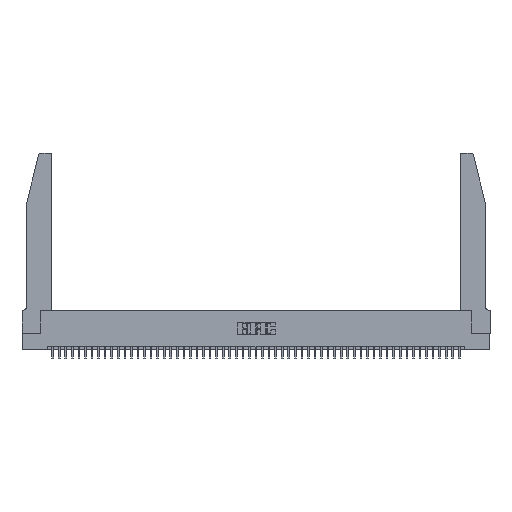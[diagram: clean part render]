
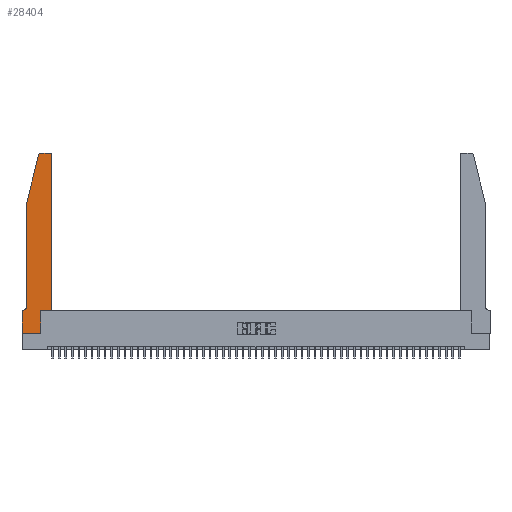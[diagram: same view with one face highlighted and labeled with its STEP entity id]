
A CAD part, top view. The second image highlights one B-rep face of the part: STEP entity #28404.
In plain terms, the highlighted planar face has unit normal (0, 0, 1).
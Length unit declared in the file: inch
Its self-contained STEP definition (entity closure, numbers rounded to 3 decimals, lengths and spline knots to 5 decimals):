
#653 = AXIS2_PLACEMENT_3D ( 'NONE', #5602, #33332, #9619 ) ;
#701 = CIRCLE ( 'NONE', #653, 0.03 ) ;
#879 = VERTEX_POINT ( 'NONE', #44375 ) ;
#1047 = DIRECTION ( 'NONE',  ( 0., -1., 0. ) ) ;
#1328 = VERTEX_POINT ( 'NONE', #31188 ) ;
#2118 = VERTEX_POINT ( 'NONE', #18137 ) ;
#2484 = CARTESIAN_POINT ( 'NONE',  ( 0.0755, 0.42, 0.37 ) ) ;
#4215 = CARTESIAN_POINT ( 'NONE',  ( 0.4205, 2.75, 0.37 ) ) ;
#4865 = CARTESIAN_POINT ( 'NONE',  ( 0., 0., 0.37 ) ) ;
#5602 = CARTESIAN_POINT ( 'NONE',  ( 0.284, 2.72, 0.37 ) ) ;
#5902 = ORIENTED_EDGE ( 'NONE', *, *, #31229, .T. ) ;
#6054 = ORIENTED_EDGE ( 'NONE', *, *, #18705, .T. ) ;
#6133 = VECTOR ( 'NONE', #19532, 39.37008 ) ;
#6512 = DIRECTION ( 'NONE',  ( 0., -1., 0. ) ) ;
#6820 = CARTESIAN_POINT ( 'NONE',  ( 0.4505, 0.35, 0.37 ) ) ;
#6958 = EDGE_CURVE ( 'NONE', #16118, #26908, #17446, .T. ) ;
#7067 = PLANE ( 'NONE',  #27129 ) ;
#7521 = DIRECTION ( 'NONE',  ( -0.239, -0.971, 0. ) ) ;
#7582 = CARTESIAN_POINT ( 'NONE',  ( 0.2865, 0.35, 0.37 ) ) ;
#9176 = ORIENTED_EDGE ( 'NONE', *, *, #27044, .T. ) ;
#9241 = VECTOR ( 'NONE', #47146, 39.37008 ) ;
#9619 = DIRECTION ( 'NONE',  ( 1., 0., 0. ) ) ;
#9884 = LINE ( 'NONE', #42937, #9241 ) ;
#10325 = LINE ( 'NONE', #6820, #22086 ) ;
#10502 = AXIS2_PLACEMENT_3D ( 'NONE', #43571, #12351, #43731 ) ;
#11084 = CARTESIAN_POINT ( 'NONE',  ( 0.25487, 2.72718, 0.37 ) ) ;
#11489 = DIRECTION ( 'NONE',  ( 1., 0., 0. ) ) ;
#12200 = LINE ( 'NONE', #18637, #21489 ) ;
#12295 = CARTESIAN_POINT ( 'NONE',  ( 0.4205, 2.72, 0.37 ) ) ;
#12351 = DIRECTION ( 'NONE',  ( 0., 0., -1. ) ) ;
#12828 = DIRECTION ( 'NONE',  ( 1., 0., 0. ) ) ;
#13343 = EDGE_CURVE ( 'NONE', #30777, #39542, #33662, .T. ) ;
#13391 = CARTESIAN_POINT ( 'NONE',  ( 0., 0.35, 0.37 ) ) ;
#14539 = ORIENTED_EDGE ( 'NONE', *, *, #36017, .T. ) ;
#15573 = EDGE_CURVE ( 'NONE', #39542, #36829, #41625, .T. ) ;
#15730 = DIRECTION ( 'NONE',  ( -1., 0., 0. ) ) ;
#16118 = VERTEX_POINT ( 'NONE', #35671 ) ;
#16507 = EDGE_LOOP ( 'NONE', ( #49306, #48106, #5902, #32633, #19754, #27828, #46066, #9176, #47113, #6054, #17876, #14539 ) ) ;
#17446 = LINE ( 'NONE', #46673, #47895 ) ;
#17876 = ORIENTED_EDGE ( 'NONE', *, *, #6958, .T. ) ;
#18137 = CARTESIAN_POINT ( 'NONE',  ( 0.2865, 0., 0.37 ) ) ;
#18637 = CARTESIAN_POINT ( 'NONE',  ( 0., 0., 0.37 ) ) ;
#18705 = EDGE_CURVE ( 'NONE', #1328, #16118, #10325, .T. ) ;
#19361 = VERTEX_POINT ( 'NONE', #4215 ) ;
#19532 = DIRECTION ( 'NONE',  ( 0., 1., 0. ) ) ;
#19754 = ORIENTED_EDGE ( 'NONE', *, *, #15573, .T. ) ;
#20386 = AXIS2_PLACEMENT_3D ( 'NONE', #12295, #28242, #12828 ) ;
#20426 = LINE ( 'NONE', #7582, #6133 ) ;
#20603 = VERTEX_POINT ( 'NONE', #11084 ) ;
#21367 = EDGE_CURVE ( 'NONE', #879, #20603, #701, .T. ) ;
#21489 = VECTOR ( 'NONE', #46227, 39.37008 ) ;
#21860 = VECTOR ( 'NONE', #7521, 39.37008 ) ;
#22086 = VECTOR ( 'NONE', #11489, 39.37008 ) ;
#22118 = CARTESIAN_POINT ( 'NONE',  ( 0.0755, 2., 0.37 ) ) ;
#23271 = CARTESIAN_POINT ( 'NONE',  ( 0., 0., 0.37 ) ) ;
#26692 = CIRCLE ( 'NONE', #20386, 0.03 ) ;
#26908 = VERTEX_POINT ( 'NONE', #34213 ) ;
#27044 = EDGE_CURVE ( 'NONE', #50103, #2118, #12200, .T. ) ;
#27129 = AXIS2_PLACEMENT_3D ( 'NONE', #30992, #42956, #43116 ) ;
#27828 = ORIENTED_EDGE ( 'NONE', *, *, #36453, .T. ) ;
#28167 = CARTESIAN_POINT ( 'NONE',  ( 0.2605, 2.75, 0.37 ) ) ;
#28242 = DIRECTION ( 'NONE',  ( 0., 0., 1. ) ) ;
#28404 = ADVANCED_FACE ( 'NONE', ( #48871 ), #7067, .T. ) ;
#29342 = EDGE_CURVE ( 'NONE', #29531, #50103, #49410, .T. ) ;
#29531 = VERTEX_POINT ( 'NONE', #13391 ) ;
#30435 = LINE ( 'NONE', #28167, #44046 ) ;
#30777 = VERTEX_POINT ( 'NONE', #32677 ) ;
#30992 = CARTESIAN_POINT ( 'NONE',  ( 0., 0.35, 0.37 ) ) ;
#31188 = CARTESIAN_POINT ( 'NONE',  ( 0.2865, 0.35, 0.37 ) ) ;
#31229 = EDGE_CURVE ( 'NONE', #20603, #30777, #40434, .T. ) ;
#31773 = CARTESIAN_POINT ( 'NONE',  ( 0.0755, 2., 0.37 ) ) ;
#32156 = CARTESIAN_POINT ( 'NONE',  ( 0.0055, 0.35, 0.37 ) ) ;
#32633 = ORIENTED_EDGE ( 'NONE', *, *, #13343, .T. ) ;
#32677 = CARTESIAN_POINT ( 'NONE',  ( 0.0755, 2., 0.37 ) ) ;
#33332 = DIRECTION ( 'NONE',  ( 0., 0., 1. ) ) ;
#33662 = LINE ( 'NONE', #22118, #39846 ) ;
#34213 = CARTESIAN_POINT ( 'NONE',  ( 0.4505, 2.72, 0.37 ) ) ;
#35671 = CARTESIAN_POINT ( 'NONE',  ( 0.4505, 0.35, 0.37 ) ) ;
#36017 = EDGE_CURVE ( 'NONE', #26908, #19361, #26692, .T. ) ;
#36453 = EDGE_CURVE ( 'NONE', #36829, #29531, #9884, .T. ) ;
#36682 = EDGE_CURVE ( 'NONE', #2118, #1328, #20426, .T. ) ;
#36829 = VERTEX_POINT ( 'NONE', #32156 ) ;
#39542 = VERTEX_POINT ( 'NONE', #2484 ) ;
#39846 = VECTOR ( 'NONE', #6512, 39.37008 ) ;
#40434 = LINE ( 'NONE', #31773, #21860 ) ;
#41625 = CIRCLE ( 'NONE', #10502, 0.07 ) ;
#42937 = CARTESIAN_POINT ( 'NONE',  ( 0.0755, 0.35, 0.37 ) ) ;
#42956 = DIRECTION ( 'NONE',  ( 0., 0., 1. ) ) ;
#43116 = DIRECTION ( 'NONE',  ( 1., 0., 0. ) ) ;
#43456 = EDGE_CURVE ( 'NONE', #19361, #879, #30435, .T. ) ;
#43571 = CARTESIAN_POINT ( 'NONE',  ( 0.0055, 0.42, 0.37 ) ) ;
#43731 = DIRECTION ( 'NONE',  ( -1., 0., 0. ) ) ;
#44046 = VECTOR ( 'NONE', #15730, 39.37008 ) ;
#44375 = CARTESIAN_POINT ( 'NONE',  ( 0.284, 2.75, 0.37 ) ) ;
#46066 = ORIENTED_EDGE ( 'NONE', *, *, #29342, .T. ) ;
#46227 = DIRECTION ( 'NONE',  ( 1., 0., 0. ) ) ;
#46673 = CARTESIAN_POINT ( 'NONE',  ( 0.4505, 0.35, 0.37 ) ) ;
#47113 = ORIENTED_EDGE ( 'NONE', *, *, #36682, .T. ) ;
#47146 = DIRECTION ( 'NONE',  ( -1., 0., 0. ) ) ;
#47895 = VECTOR ( 'NONE', #51147, 39.37008 ) ;
#48106 = ORIENTED_EDGE ( 'NONE', *, *, #21367, .T. ) ;
#48176 = VECTOR ( 'NONE', #1047, 39.37008 ) ;
#48871 = FACE_OUTER_BOUND ( 'NONE', #16507, .T. ) ;
#49306 = ORIENTED_EDGE ( 'NONE', *, *, #43456, .T. ) ;
#49410 = LINE ( 'NONE', #4865, #48176 ) ;
#50103 = VERTEX_POINT ( 'NONE', #23271 ) ;
#51147 = DIRECTION ( 'NONE',  ( 0., 1., 0. ) ) ;
